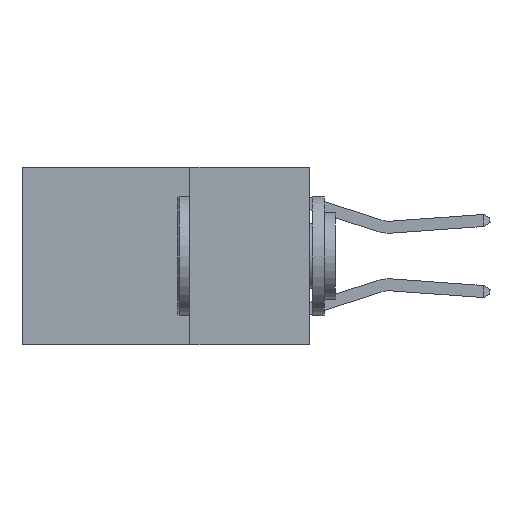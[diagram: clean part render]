
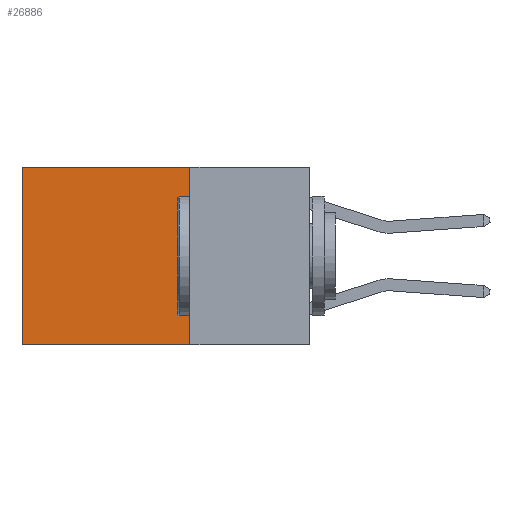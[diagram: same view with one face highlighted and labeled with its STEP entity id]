
A CAD part, left-side view. The second image highlights one B-rep face of the part: STEP entity #26886.
In plain terms, the highlighted planar face has unit normal (-1, 0, 0).
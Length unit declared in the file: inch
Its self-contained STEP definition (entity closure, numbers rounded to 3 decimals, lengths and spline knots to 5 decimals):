
#2174 = FACE_OUTER_BOUND ( 'NONE', #20615, .T. ) ;
#2361 = LINE ( 'NONE', #6797, #29195 ) ;
#2481 = DIRECTION ( 'NONE',  ( 0., 0., -1. ) ) ;
#2551 = VECTOR ( 'NONE', #21038, 39.37008 ) ;
#2748 = EDGE_CURVE ( 'NONE', #26193, #18891, #3547, .T. ) ;
#2837 = CARTESIAN_POINT ( 'NONE',  ( 0.2625, 0.25, -0.37 ) ) ;
#3547 = LINE ( 'NONE', #10525, #24051 ) ;
#4103 = VERTEX_POINT ( 'NONE', #21476 ) ;
#4635 = CARTESIAN_POINT ( 'NONE',  ( 0.2625, 0.25, 0. ) ) ;
#6296 = ORIENTED_EDGE ( 'NONE', *, *, #8771, .T. ) ;
#6703 = CARTESIAN_POINT ( 'NONE',  ( 0.2625, 0.6, 0. ) ) ;
#6797 = CARTESIAN_POINT ( 'NONE',  ( 0.2625, 0.25, 0. ) ) ;
#8771 = EDGE_CURVE ( 'NONE', #26193, #4103, #2361, .T. ) ;
#10525 = CARTESIAN_POINT ( 'NONE',  ( 0.2625, 0.25, 0. ) ) ;
#11196 = ORIENTED_EDGE ( 'NONE', *, *, #2748, .F. ) ;
#11917 = CARTESIAN_POINT ( 'NONE',  ( 0.2625, 0.25, -0.37 ) ) ;
#11938 = VERTEX_POINT ( 'NONE', #19507 ) ;
#13643 = EDGE_CURVE ( 'NONE', #4103, #11938, #27522, .T. ) ;
#14263 = EDGE_CURVE ( 'NONE', #18891, #11938, #25950, .T. ) ;
#15922 = DIRECTION ( 'NONE',  ( 1., 0., 0. ) ) ;
#18891 = VERTEX_POINT ( 'NONE', #11917 ) ;
#19023 = DIRECTION ( 'NONE',  ( 0., 1., 0. ) ) ;
#19085 = AXIS2_PLACEMENT_3D ( 'NONE', #4635, #15922, #2481 ) ;
#19507 = CARTESIAN_POINT ( 'NONE',  ( 0.2625, 0.6, -0.37 ) ) ;
#20482 = PLANE ( 'NONE',  #19085 ) ;
#20615 = EDGE_LOOP ( 'NONE', ( #20856, #29253, #11196, #6296 ) ) ;
#20856 = ORIENTED_EDGE ( 'NONE', *, *, #13643, .T. ) ;
#21038 = DIRECTION ( 'NONE',  ( 0., 0., -1. ) ) ;
#21476 = CARTESIAN_POINT ( 'NONE',  ( 0.2625, 0.6, 0. ) ) ;
#22991 = DIRECTION ( 'NONE',  ( 0., 1., 0. ) ) ;
#24051 = VECTOR ( 'NONE', #24640, 39.37008 ) ;
#24261 = CARTESIAN_POINT ( 'NONE',  ( 0.2625, 0.25, 0. ) ) ;
#24640 = DIRECTION ( 'NONE',  ( 0., 0., -1. ) ) ;
#25950 = LINE ( 'NONE', #2837, #28259 ) ;
#26193 = VERTEX_POINT ( 'NONE', #24261 ) ;
#26886 = ADVANCED_FACE ( 'NONE', ( #2174 ), #20482, .F. ) ;
#27522 = LINE ( 'NONE', #6703, #2551 ) ;
#28259 = VECTOR ( 'NONE', #19023, 39.37008 ) ;
#29195 = VECTOR ( 'NONE', #22991, 39.37008 ) ;
#29253 = ORIENTED_EDGE ( 'NONE', *, *, #14263, .F. ) ;
